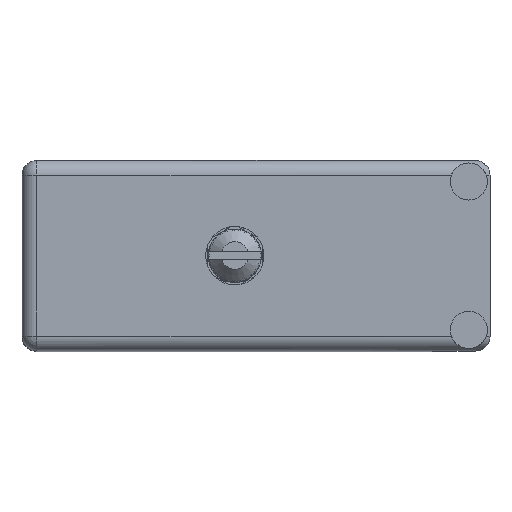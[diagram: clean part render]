
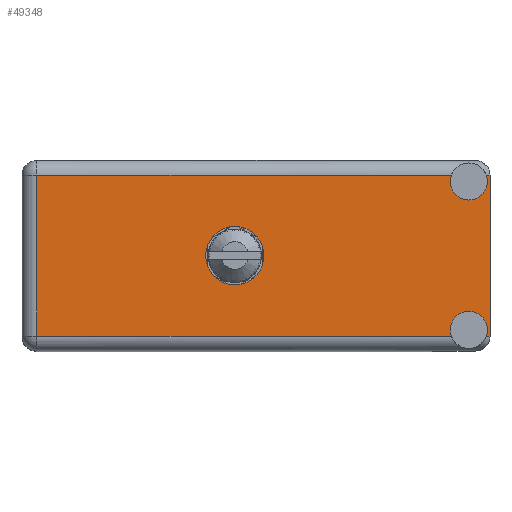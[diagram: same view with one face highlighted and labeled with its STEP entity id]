
A CAD part, top view. The second image highlights one B-rep face of the part: STEP entity #49348.
In plain terms, the highlighted face is planar.
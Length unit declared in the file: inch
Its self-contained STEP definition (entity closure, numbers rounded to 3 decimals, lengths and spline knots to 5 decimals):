
#2197 = VERTEX_POINT ( 'NONE', #11942 ) ;
#3666 = DIRECTION ( 'NONE',  ( -1., 0., 0. ) ) ;
#4342 = LINE ( 'NONE', #62996, #50585 ) ;
#4990 = VERTEX_POINT ( 'NONE', #83263 ) ;
#5391 = VERTEX_POINT ( 'NONE', #53158 ) ;
#5904 = CIRCLE ( 'NONE', #84344, 0.1375 ) ;
#6747 = DIRECTION ( 'NONE',  ( 0., 0., 1. ) ) ;
#11942 = CARTESIAN_POINT ( 'NONE',  ( 2.19038, 1.566, -0.829 ) ) ;
#13995 = ORIENTED_EDGE ( 'NONE', *, *, #99591, .T. ) ;
#16953 = ORIENTED_EDGE ( 'NONE', *, *, #99693, .F. ) ;
#17979 = DIRECTION ( 'NONE',  ( 0., 1., 0. ) ) ;
#19474 = CARTESIAN_POINT ( 'NONE',  ( 0., 1.566, -0.829 ) ) ;
#19945 = ORIENTED_EDGE ( 'NONE', *, *, #74268, .T. ) ;
#20322 = DIRECTION ( 'NONE',  ( 1., 0., 0. ) ) ;
#21555 = VERTEX_POINT ( 'NONE', #99329 ) ;
#22243 = EDGE_LOOP ( 'NONE', ( #16953, #25201 ) ) ;
#24136 = AXIS2_PLACEMENT_3D ( 'NONE', #59326, #100850, #91489 ) ;
#25201 = ORIENTED_EDGE ( 'NONE', *, *, #80670, .F. ) ;
#25648 = EDGE_CURVE ( 'NONE', #103693, #5391, #4342, .T. ) ;
#26479 = EDGE_CURVE ( 'NONE', #5391, #21555, #106083, .T. ) ;
#26500 = CARTESIAN_POINT ( 'NONE',  ( 2.208, 1.566, -0.07 ) ) ;
#26903 = CARTESIAN_POINT ( 'NONE',  ( 2.108, 1.566, -0.0995 ) ) ;
#27256 = AXIS2_PLACEMENT_3D ( 'NONE', #26903, #59196, #84096 ) ;
#27780 = CIRCLE ( 'NONE', #86007, 0.1375 ) ;
#29425 = LINE ( 'NONE', #91696, #34602 ) ;
#30499 = DIRECTION ( 'NONE',  ( 0., 0., 1. ) ) ;
#30507 = DIRECTION ( 'NONE',  ( 0., 0., 1. ) ) ;
#30851 = DIRECTION ( 'NONE',  ( 0., 1., 0. ) ) ;
#30872 = CARTESIAN_POINT ( 'NONE',  ( 2.108, 1.566, -0.7995 ) ) ;
#32740 = CARTESIAN_POINT ( 'NONE',  ( 2.02562, 1.566, -0.829 ) ) ;
#33697 = EDGE_CURVE ( 'NONE', #67557, #21555, #46563, .T. ) ;
#34471 = DIRECTION ( 'NONE',  ( 1., 0., 0. ) ) ;
#34602 = VECTOR ( 'NONE', #34471, 39.37008 ) ;
#39895 = ORIENTED_EDGE ( 'NONE', *, *, #98342, .F. ) ;
#41363 = EDGE_LOOP ( 'NONE', ( #50956, #58711, #56799, #98381, #41620, #13995, #86906, #39895, #19945, #41498 ) ) ;
#41498 = ORIENTED_EDGE ( 'NONE', *, *, #25648, .T. ) ;
#41620 = ORIENTED_EDGE ( 'NONE', *, *, #91026, .F. ) ;
#42376 = EDGE_CURVE ( 'NONE', #4990, #2197, #69762, .T. ) ;
#42901 = CARTESIAN_POINT ( 'NONE',  ( 2.208, 1.566, 0. ) ) ;
#43508 = DIRECTION ( 'NONE',  ( 0., 0., 1. ) ) ;
#45059 = CARTESIAN_POINT ( 'NONE',  ( 0.07, 1.566, -0.829 ) ) ;
#45199 = VERTEX_POINT ( 'NONE', #87464 ) ;
#45253 = VERTEX_POINT ( 'NONE', #32740 ) ;
#46182 = VERTEX_POINT ( 'NONE', #57077 ) ;
#46563 = CIRCLE ( 'NONE', #24136, 0.0875 ) ;
#46648 = CARTESIAN_POINT ( 'NONE',  ( 2.108, 1.566, -0.7995 ) ) ;
#46660 = DIRECTION ( 'NONE',  ( 0., 1., 0. ) ) ;
#48084 = DIRECTION ( 'NONE',  ( 0., 0., 1. ) ) ;
#49348 = ADVANCED_FACE ( 'NONE', ( #71190, #53188 ), #96050, .T. ) ;
#49389 = VECTOR ( 'NONE', #3666, 39.37008 ) ;
#49713 = CARTESIAN_POINT ( 'NONE',  ( 2.108, 1.566, -0.187 ) ) ;
#49791 = CARTESIAN_POINT ( 'NONE',  ( 1.004, 1.566, -0.587 ) ) ;
#50585 = VECTOR ( 'NONE', #77386, 39.37008 ) ;
#50956 = ORIENTED_EDGE ( 'NONE', *, *, #26479, .T. ) ;
#53158 = CARTESIAN_POINT ( 'NONE',  ( 0.07, 1.566, -0.07 ) ) ;
#53188 = FACE_OUTER_BOUND ( 'NONE', #41363, .T. ) ;
#56799 = ORIENTED_EDGE ( 'NONE', *, *, #57375, .F. ) ;
#57077 = CARTESIAN_POINT ( 'NONE',  ( 2.208, 1.566, -0.07 ) ) ;
#57375 = EDGE_CURVE ( 'NONE', #106787, #67557, #87562, .T. ) ;
#58625 = VERTEX_POINT ( 'NONE', #70520 ) ;
#58711 = ORIENTED_EDGE ( 'NONE', *, *, #33697, .F. ) ;
#59196 = DIRECTION ( 'NONE',  ( 0., 1., 0. ) ) ;
#59326 = CARTESIAN_POINT ( 'NONE',  ( 2.108, 1.566, -0.0995 ) ) ;
#62825 = AXIS2_PLACEMENT_3D ( 'NONE', #46648, #30851, #30499 ) ;
#62996 = CARTESIAN_POINT ( 'NONE',  ( 0.07, 1.566, -0.899 ) ) ;
#63815 = LINE ( 'NONE', #42901, #85722 ) ;
#67557 = VERTEX_POINT ( 'NONE', #49713 ) ;
#69546 = VERTEX_POINT ( 'NONE', #49791 ) ;
#69762 = CIRCLE ( 'NONE', #62825, 0.0875 ) ;
#70520 = CARTESIAN_POINT ( 'NONE',  ( 1.004, 1.566, -0.312 ) ) ;
#71190 = FACE_BOUND ( 'NONE', #22243, .T. ) ;
#72223 = CARTESIAN_POINT ( 'NONE',  ( 2.19038, 1.566, -0.07 ) ) ;
#73417 = CARTESIAN_POINT ( 'NONE',  ( 0., 1.566, -0.829 ) ) ;
#74268 = EDGE_CURVE ( 'NONE', #45253, #103693, #76255, .T. ) ;
#76154 = EDGE_CURVE ( 'NONE', #106787, #46182, #29425, .T. ) ;
#76255 = LINE ( 'NONE', #19474, #49389 ) ;
#77386 = DIRECTION ( 'NONE',  ( 0., 0., 1. ) ) ;
#80670 = EDGE_CURVE ( 'NONE', #69546, #58625, #5904, .T. ) ;
#80671 = VECTOR ( 'NONE', #90069, 39.37008 ) ;
#83263 = CARTESIAN_POINT ( 'NONE',  ( 2.108, 1.566, -0.712 ) ) ;
#84096 = DIRECTION ( 'NONE',  ( 0., 0., 1. ) ) ;
#84344 = AXIS2_PLACEMENT_3D ( 'NONE', #90919, #97470, #48084 ) ;
#85722 = VECTOR ( 'NONE', #94780, 39.37008 ) ;
#86007 = AXIS2_PLACEMENT_3D ( 'NONE', #93243, #17979, #43508 ) ;
#86033 = CIRCLE ( 'NONE', #99631, 0.0875 ) ;
#86906 = ORIENTED_EDGE ( 'NONE', *, *, #42376, .F. ) ;
#87464 = CARTESIAN_POINT ( 'NONE',  ( 2.208, 1.566, -0.829 ) ) ;
#87562 = CIRCLE ( 'NONE', #27256, 0.0875 ) ;
#90069 = DIRECTION ( 'NONE',  ( -1., 0., 0. ) ) ;
#90919 = CARTESIAN_POINT ( 'NONE',  ( 1.004, 1.566, -0.4495 ) ) ;
#91026 = EDGE_CURVE ( 'NONE', #45199, #46182, #63815, .T. ) ;
#91489 = DIRECTION ( 'NONE',  ( 0., 0., 1. ) ) ;
#91696 = CARTESIAN_POINT ( 'NONE',  ( 2.208, 1.566, -0.07 ) ) ;
#93243 = CARTESIAN_POINT ( 'NONE',  ( 1.004, 1.566, -0.4495 ) ) ;
#94780 = DIRECTION ( 'NONE',  ( 0., 0., 1. ) ) ;
#95421 = AXIS2_PLACEMENT_3D ( 'NONE', #105333, #46660, #30507 ) ;
#96050 = PLANE ( 'NONE',  #95421 ) ;
#97470 = DIRECTION ( 'NONE',  ( 0., 1., 0. ) ) ;
#97817 = DIRECTION ( 'NONE',  ( 0., 1., 0. ) ) ;
#98342 = EDGE_CURVE ( 'NONE', #45253, #4990, #86033, .T. ) ;
#98381 = ORIENTED_EDGE ( 'NONE', *, *, #76154, .T. ) ;
#99329 = CARTESIAN_POINT ( 'NONE',  ( 2.02562, 1.566, -0.07 ) ) ;
#99591 = EDGE_CURVE ( 'NONE', #45199, #2197, #102618, .T. ) ;
#99631 = AXIS2_PLACEMENT_3D ( 'NONE', #30872, #97817, #6747 ) ;
#99693 = EDGE_CURVE ( 'NONE', #58625, #69546, #27780, .T. ) ;
#99714 = VECTOR ( 'NONE', #20322, 39.37008 ) ;
#100850 = DIRECTION ( 'NONE',  ( 0., 1., 0. ) ) ;
#102618 = LINE ( 'NONE', #73417, #80671 ) ;
#103693 = VERTEX_POINT ( 'NONE', #45059 ) ;
#105333 = CARTESIAN_POINT ( 'NONE',  ( 0., 1.566, -0.899 ) ) ;
#106083 = LINE ( 'NONE', #26500, #99714 ) ;
#106787 = VERTEX_POINT ( 'NONE', #72223 ) ;
